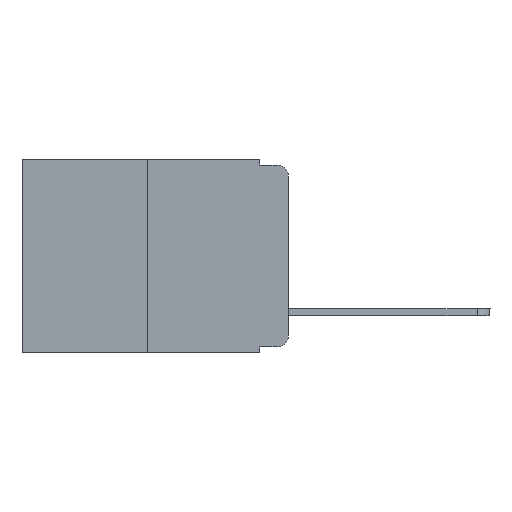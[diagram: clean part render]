
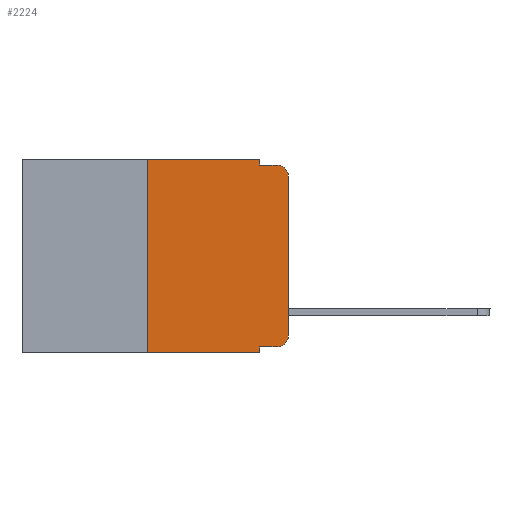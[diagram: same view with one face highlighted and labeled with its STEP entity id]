
A CAD part, left-side view. The second image highlights one B-rep face of the part: STEP entity #2224.
In plain terms, the highlighted planar face has unit normal (-1, 0, 0).
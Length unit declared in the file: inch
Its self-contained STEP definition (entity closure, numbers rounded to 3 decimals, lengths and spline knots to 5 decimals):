
#217 = ORIENTED_EDGE ( 'NONE', *, *, #7450, .F. ) ;
#363 = DIRECTION ( 'NONE',  ( 0., 0., -1. ) ) ;
#671 = CARTESIAN_POINT ( 'NONE',  ( 0., 0., -0.03 ) ) ;
#797 = CARTESIAN_POINT ( 'NONE',  ( 0., 0.051, 0. ) ) ;
#810 = VERTEX_POINT ( 'NONE', #2587 ) ;
#840 = DIRECTION ( 'NONE',  ( 0., -1., 0. ) ) ;
#852 = CIRCLE ( 'NONE', #4850, 0.02 ) ;
#944 = EDGE_CURVE ( 'NONE', #810, #7157, #3564, .T. ) ;
#982 = DIRECTION ( 'NONE',  ( 1., 0., 0. ) ) ;
#1458 = VECTOR ( 'NONE', #2236, 39.37008 ) ;
#1729 = LINE ( 'NONE', #9707, #7123 ) ;
#1758 = VERTEX_POINT ( 'NONE', #9488 ) ;
#2014 = EDGE_LOOP ( 'NONE', ( #4951, #4142, #10444, #2103, #4991, #217, #5714, #5922, #2896, #6945 ) ) ;
#2103 = ORIENTED_EDGE ( 'NONE', *, *, #10597, .F. ) ;
#2172 = VECTOR ( 'NONE', #10543, 39.37008 ) ;
#2224 = ADVANCED_FACE ( 'NONE', ( #12753 ), #7897, .F. ) ;
#2236 = DIRECTION ( 'NONE',  ( 0., -1., 0. ) ) ;
#2587 = CARTESIAN_POINT ( 'NONE',  ( 0., 0., -0.313 ) ) ;
#2618 = AXIS2_PLACEMENT_3D ( 'NONE', #5002, #982, #10929 ) ;
#2896 = ORIENTED_EDGE ( 'NONE', *, *, #6597, .T. ) ;
#2995 = DIRECTION ( 'NONE',  ( 0., -1., 0. ) ) ;
#3127 = LINE ( 'NONE', #8960, #3177 ) ;
#3177 = VECTOR ( 'NONE', #2995, 39.37008 ) ;
#3198 = CARTESIAN_POINT ( 'NONE',  ( 0., 0.051, -0.01 ) ) ;
#3564 = LINE ( 'NONE', #7578, #11569 ) ;
#3696 = DIRECTION ( 'NONE',  ( 0., 0., 1. ) ) ;
#3742 = VECTOR ( 'NONE', #363, 39.37008 ) ;
#3931 = DIRECTION ( 'NONE',  ( 0., 0., -1. ) ) ;
#4142 = ORIENTED_EDGE ( 'NONE', *, *, #5535, .T. ) ;
#4565 = DIRECTION ( 'NONE',  ( -1., 0., 0. ) ) ;
#4585 = EDGE_CURVE ( 'NONE', #8919, #11506, #11025, .T. ) ;
#4826 = LINE ( 'NONE', #797, #9453 ) ;
#4831 = VERTEX_POINT ( 'NONE', #8811 ) ;
#4850 = AXIS2_PLACEMENT_3D ( 'NONE', #7805, #8060, #3931 ) ;
#4951 = ORIENTED_EDGE ( 'NONE', *, *, #944, .T. ) ;
#4991 = ORIENTED_EDGE ( 'NONE', *, *, #6300, .F. ) ;
#5002 = CARTESIAN_POINT ( 'NONE',  ( 0., 0.473, 0. ) ) ;
#5468 = CARTESIAN_POINT ( 'NONE',  ( 0., 0.051, 0. ) ) ;
#5535 = EDGE_CURVE ( 'NONE', #7157, #11506, #852, .T. ) ;
#5714 = ORIENTED_EDGE ( 'NONE', *, *, #10448, .T. ) ;
#5759 = EDGE_CURVE ( 'NONE', #10695, #9531, #4826, .T. ) ;
#5922 = ORIENTED_EDGE ( 'NONE', *, *, #5759, .F. ) ;
#6300 = EDGE_CURVE ( 'NONE', #8627, #12692, #1729, .T. ) ;
#6518 = VECTOR ( 'NONE', #9562, 39.37008 ) ;
#6527 = DIRECTION ( 'NONE',  ( 0., 0., -1. ) ) ;
#6597 = EDGE_CURVE ( 'NONE', #10695, #4831, #11519, .T. ) ;
#6945 = ORIENTED_EDGE ( 'NONE', *, *, #11011, .T. ) ;
#7123 = VECTOR ( 'NONE', #840, 39.37008 ) ;
#7157 = VERTEX_POINT ( 'NONE', #671 ) ;
#7450 = EDGE_CURVE ( 'NONE', #1758, #8627, #8539, .T. ) ;
#7470 = LINE ( 'NONE', #8501, #3742 ) ;
#7578 = CARTESIAN_POINT ( 'NONE',  ( 0., 0., 0. ) ) ;
#7805 = CARTESIAN_POINT ( 'NONE',  ( 0., 0.02, -0.03 ) ) ;
#7820 = CARTESIAN_POINT ( 'NONE',  ( 0., 0.02, -0.01 ) ) ;
#7897 = PLANE ( 'NONE',  #2618 ) ;
#7912 = DIRECTION ( 'NONE',  ( 0., 0., -1. ) ) ;
#8060 = DIRECTION ( 'NONE',  ( -1., 0., 0. ) ) ;
#8420 = AXIS2_PLACEMENT_3D ( 'NONE', #12324, #4565, #6527 ) ;
#8501 = CARTESIAN_POINT ( 'NONE',  ( 0., 0.051, 0. ) ) ;
#8539 = LINE ( 'NONE', #11541, #2172 ) ;
#8627 = VERTEX_POINT ( 'NONE', #8891 ) ;
#8811 = CARTESIAN_POINT ( 'NONE',  ( 0., 0.02, -0.333 ) ) ;
#8891 = CARTESIAN_POINT ( 'NONE',  ( 0., 0.25, 0. ) ) ;
#8919 = VERTEX_POINT ( 'NONE', #12835 ) ;
#8960 = CARTESIAN_POINT ( 'NONE',  ( 0., 0.473, -0.343 ) ) ;
#9307 = CARTESIAN_POINT ( 'NONE',  ( 0., 0.051, -0.343 ) ) ;
#9453 = VECTOR ( 'NONE', #7912, 39.37008 ) ;
#9488 = CARTESIAN_POINT ( 'NONE',  ( 0., 0.25, -0.343 ) ) ;
#9531 = VERTEX_POINT ( 'NONE', #9307 ) ;
#9562 = DIRECTION ( 'NONE',  ( 0., -1., 0. ) ) ;
#9707 = CARTESIAN_POINT ( 'NONE',  ( 0., 0.473, 0. ) ) ;
#10444 = ORIENTED_EDGE ( 'NONE', *, *, #4585, .F. ) ;
#10448 = EDGE_CURVE ( 'NONE', #1758, #9531, #3127, .T. ) ;
#10543 = DIRECTION ( 'NONE',  ( 0., 0., 1. ) ) ;
#10587 = CARTESIAN_POINT ( 'NONE',  ( 0., 0.051, -0.333 ) ) ;
#10597 = EDGE_CURVE ( 'NONE', #12692, #8919, #7470, .T. ) ;
#10695 = VERTEX_POINT ( 'NONE', #11870 ) ;
#10929 = DIRECTION ( 'NONE',  ( 0., 0., -1. ) ) ;
#11011 = EDGE_CURVE ( 'NONE', #4831, #810, #12364, .T. ) ;
#11025 = LINE ( 'NONE', #3198, #1458 ) ;
#11506 = VERTEX_POINT ( 'NONE', #7820 ) ;
#11519 = LINE ( 'NONE', #10587, #6518 ) ;
#11541 = CARTESIAN_POINT ( 'NONE',  ( 0., 0.25, 0. ) ) ;
#11569 = VECTOR ( 'NONE', #3696, 39.37008 ) ;
#11870 = CARTESIAN_POINT ( 'NONE',  ( 0., 0.051, -0.333 ) ) ;
#12324 = CARTESIAN_POINT ( 'NONE',  ( 0., 0.02, -0.313 ) ) ;
#12364 = CIRCLE ( 'NONE', #8420, 0.02 ) ;
#12692 = VERTEX_POINT ( 'NONE', #5468 ) ;
#12753 = FACE_OUTER_BOUND ( 'NONE', #2014, .T. ) ;
#12835 = CARTESIAN_POINT ( 'NONE',  ( 0., 0.051, -0.01 ) ) ;
